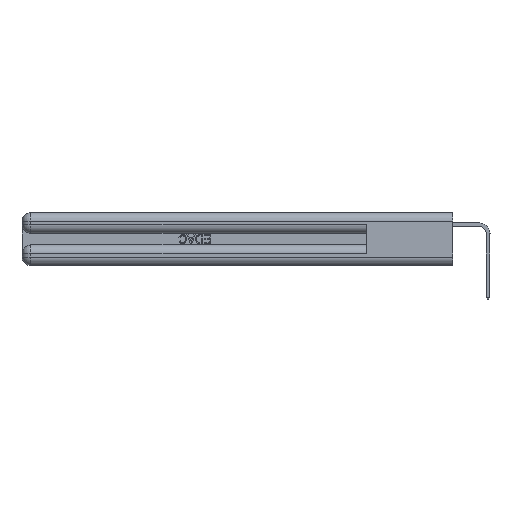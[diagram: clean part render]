
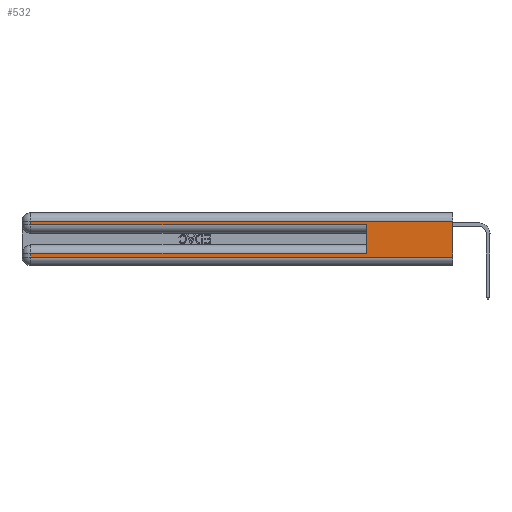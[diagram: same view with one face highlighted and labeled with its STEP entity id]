
A CAD part, left-side view. The second image highlights one B-rep face of the part: STEP entity #532.
In plain terms, the highlighted planar face has unit normal (-1, 0, 0).
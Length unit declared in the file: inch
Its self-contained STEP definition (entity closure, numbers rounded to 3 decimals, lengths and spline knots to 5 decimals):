
#135 = EDGE_CURVE ( 'NONE', #19695, #26029, #11710, .T. ) ;
#532 = ADVANCED_FACE ( 'NONE', ( #4068 ), #37040, .F. ) ;
#1688 = EDGE_CURVE ( 'NONE', #32533, #22073, #29246, .T. ) ;
#2130 = DIRECTION ( 'NONE',  ( 1., 0., 0. ) ) ;
#2874 = CARTESIAN_POINT ( 'NONE',  ( 0., 0.6, 0.145 ) ) ;
#3074 = CARTESIAN_POINT ( 'NONE',  ( 0., 2.94, 0.37 ) ) ;
#3292 = ORIENTED_EDGE ( 'NONE', *, *, #22083, .F. ) ;
#4068 = FACE_OUTER_BOUND ( 'NONE', #19213, .T. ) ;
#4268 = CARTESIAN_POINT ( 'NONE',  ( 0., 2.94, 0.31 ) ) ;
#4948 = VERTEX_POINT ( 'NONE', #17868 ) ;
#4999 = CARTESIAN_POINT ( 'NONE',  ( 0., 0., 0.31 ) ) ;
#6293 = DIRECTION ( 'NONE',  ( 0., 0., -1. ) ) ;
#8090 = VERTEX_POINT ( 'NONE', #21265 ) ;
#8161 = VECTOR ( 'NONE', #28597, 39.37008 ) ;
#8624 = CARTESIAN_POINT ( 'NONE',  ( 0., 2.94, 0.085 ) ) ;
#9844 = CARTESIAN_POINT ( 'NONE',  ( 0., 2.94, 0.37 ) ) ;
#10261 = EDGE_CURVE ( 'NONE', #22947, #14019, #19914, .T. ) ;
#10501 = EDGE_CURVE ( 'NONE', #4948, #22073, #15985, .T. ) ;
#11225 = CARTESIAN_POINT ( 'NONE',  ( 0., 0., 0.285 ) ) ;
#11710 = LINE ( 'NONE', #9844, #13413 ) ;
#11838 = CARTESIAN_POINT ( 'NONE',  ( 0., 0., 0.37 ) ) ;
#13413 = VECTOR ( 'NONE', #19669, 39.37008 ) ;
#14019 = VERTEX_POINT ( 'NONE', #8624 ) ;
#15926 = VECTOR ( 'NONE', #23384, 39.37008 ) ;
#15985 = LINE ( 'NONE', #16958, #15926 ) ;
#16942 = EDGE_CURVE ( 'NONE', #32533, #19695, #22562, .T. ) ;
#16958 = CARTESIAN_POINT ( 'NONE',  ( 0., 0., 0.06 ) ) ;
#17417 = VECTOR ( 'NONE', #39630, 39.37008 ) ;
#17868 = CARTESIAN_POINT ( 'NONE',  ( 0., 2.94, 0.06 ) ) ;
#17956 = LINE ( 'NONE', #2874, #8161 ) ;
#18078 = CARTESIAN_POINT ( 'NONE',  ( 0., 0.6, 0.085 ) ) ;
#19125 = ORIENTED_EDGE ( 'NONE', *, *, #10261, .T. ) ;
#19213 = EDGE_LOOP ( 'NONE', ( #37881, #35738, #37823, #20938, #3292, #19125, #21570, #27130 ) ) ;
#19669 = DIRECTION ( 'NONE',  ( 0., 0., -1. ) ) ;
#19695 = VERTEX_POINT ( 'NONE', #4268 ) ;
#19906 = VECTOR ( 'NONE', #40828, 39.37008 ) ;
#19914 = LINE ( 'NONE', #25258, #19906 ) ;
#20938 = ORIENTED_EDGE ( 'NONE', *, *, #35520, .T. ) ;
#21265 = CARTESIAN_POINT ( 'NONE',  ( 0., 0.6, 0.285 ) ) ;
#21570 = ORIENTED_EDGE ( 'NONE', *, *, #40886, .T. ) ;
#21601 = AXIS2_PLACEMENT_3D ( 'NONE', #11838, #2130, #24742 ) ;
#22073 = VERTEX_POINT ( 'NONE', #37787 ) ;
#22083 = EDGE_CURVE ( 'NONE', #22947, #8090, #17956, .T. ) ;
#22278 = VECTOR ( 'NONE', #24401, 39.37008 ) ;
#22562 = LINE ( 'NONE', #4999, #22278 ) ;
#22947 = VERTEX_POINT ( 'NONE', #18078 ) ;
#23384 = DIRECTION ( 'NONE',  ( 0., -1., 0. ) ) ;
#24401 = DIRECTION ( 'NONE',  ( 0., 1., 0. ) ) ;
#24742 = DIRECTION ( 'NONE',  ( 0., 0., -1. ) ) ;
#25258 = CARTESIAN_POINT ( 'NONE',  ( 0., 0., 0.085 ) ) ;
#26029 = VERTEX_POINT ( 'NONE', #26237 ) ;
#26237 = CARTESIAN_POINT ( 'NONE',  ( 0., 2.94, 0.285 ) ) ;
#26736 = LINE ( 'NONE', #11225, #17417 ) ;
#27130 = ORIENTED_EDGE ( 'NONE', *, *, #10501, .T. ) ;
#28597 = DIRECTION ( 'NONE',  ( 0., 0., 1. ) ) ;
#28806 = VECTOR ( 'NONE', #39162, 39.37008 ) ;
#29078 = CARTESIAN_POINT ( 'NONE',  ( 0., 0., 0.31 ) ) ;
#29246 = LINE ( 'NONE', #36034, #28806 ) ;
#32533 = VERTEX_POINT ( 'NONE', #29078 ) ;
#33223 = VECTOR ( 'NONE', #6293, 39.37008 ) ;
#34203 = LINE ( 'NONE', #3074, #33223 ) ;
#35520 = EDGE_CURVE ( 'NONE', #26029, #8090, #26736, .T. ) ;
#35738 = ORIENTED_EDGE ( 'NONE', *, *, #16942, .T. ) ;
#36034 = CARTESIAN_POINT ( 'NONE',  ( 0., 0., 0.37 ) ) ;
#37040 = PLANE ( 'NONE',  #21601 ) ;
#37787 = CARTESIAN_POINT ( 'NONE',  ( 0., 0., 0.06 ) ) ;
#37823 = ORIENTED_EDGE ( 'NONE', *, *, #135, .T. ) ;
#37881 = ORIENTED_EDGE ( 'NONE', *, *, #1688, .F. ) ;
#39162 = DIRECTION ( 'NONE',  ( 0., 0., -1. ) ) ;
#39630 = DIRECTION ( 'NONE',  ( 0., -1., 0. ) ) ;
#40828 = DIRECTION ( 'NONE',  ( 0., 1., 0. ) ) ;
#40886 = EDGE_CURVE ( 'NONE', #14019, #4948, #34203, .T. ) ;
